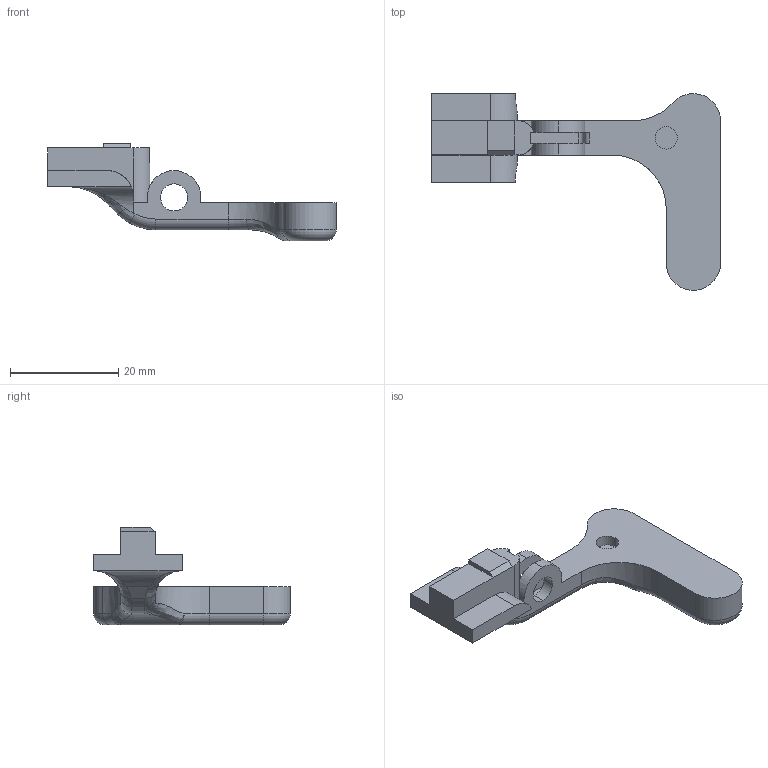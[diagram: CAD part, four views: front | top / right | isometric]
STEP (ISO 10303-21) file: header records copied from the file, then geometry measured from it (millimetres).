
FILE_DESCRIPTION (( 'STEP AP214' ), '1' );
FILE_NAME ('Kommando_rear_Release.STEP', '2013-09-01T16:43:53', ( 'Asher' ), ( '' ), 'SwSTEP 2.0', 'SolidWorks 2013', '' );
FILE_SCHEMA (( 'AUTOMOTIVE_DESIGN' ));
Length unit declared in the file: millimetre
Products named in the file (1): Kommando_rear_Release
Bounding box: 53.38 x 36.35 x 18 mm (x, y, z)
Volume: 4985.8 mm3; surface area: 3069.3 mm2
Topology: 1 solids, 1 shells, 82 faces, 208 edges, 127 vertices
Faces by surface type: plane 34, cylinder 30, bspline 8, torus 8, sphere 2
Entity records: 2763 total; most frequent: CARTESIAN_POINT 782, ORIENTED_EDGE 412, DIRECTION 409, EDGE_CURVE 206, AXIS2_PLACEMENT_3D 152, VERTEX_POINT 127, VECTOR 105, LINE 105
